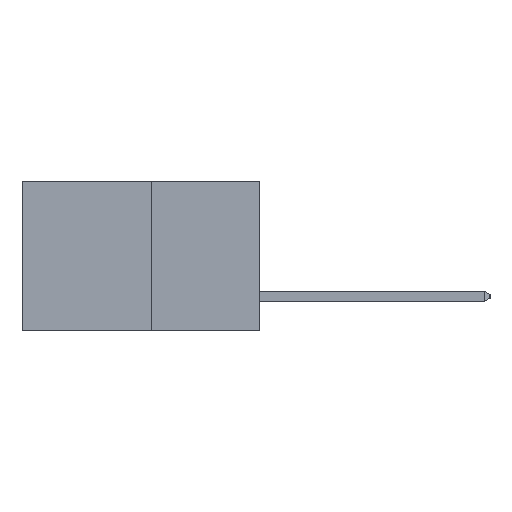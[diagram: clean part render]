
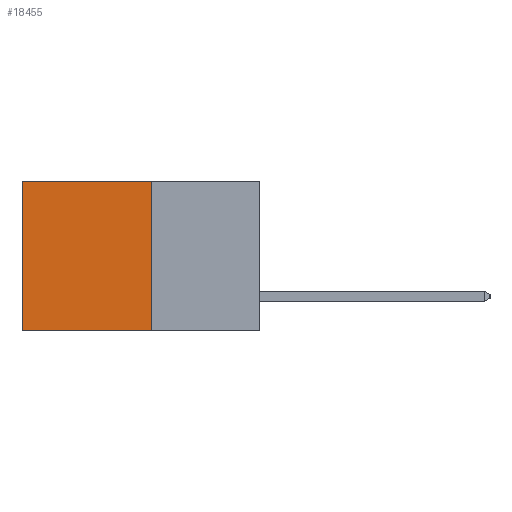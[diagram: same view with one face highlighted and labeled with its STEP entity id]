
A CAD part, left-side view. The second image highlights one B-rep face of the part: STEP entity #18455.
In plain terms, the highlighted planar face has unit normal (-1, 0, 0).
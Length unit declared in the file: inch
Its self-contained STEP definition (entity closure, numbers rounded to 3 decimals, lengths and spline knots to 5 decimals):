
#78 = ORIENTED_EDGE ( 'NONE', *, *, #591, .F. ) ;
#591 = EDGE_CURVE ( 'NONE', #16382, #14361, #10443, .T. ) ;
#1503 = FACE_OUTER_BOUND ( 'NONE', #6174, .T. ) ;
#1516 = CARTESIAN_POINT ( 'NONE',  ( 0.277, 0.27, -0.37 ) ) ;
#1697 = VECTOR ( 'NONE', #2578, 39.37008 ) ;
#2236 = DIRECTION ( 'NONE',  ( 1., 0., 0. ) ) ;
#2578 = DIRECTION ( 'NONE',  ( 0., 0., -1. ) ) ;
#2659 = VECTOR ( 'NONE', #8415, 39.37008 ) ;
#2939 = ORIENTED_EDGE ( 'NONE', *, *, #18609, .F. ) ;
#3146 = LINE ( 'NONE', #12654, #2659 ) ;
#3270 = DIRECTION ( 'NONE',  ( 0., 1., 0. ) ) ;
#3300 = VERTEX_POINT ( 'NONE', #18656 ) ;
#4979 = CARTESIAN_POINT ( 'NONE',  ( 0.277, 0.59, -0.37 ) ) ;
#6075 = LINE ( 'NONE', #18608, #1697 ) ;
#6174 = EDGE_LOOP ( 'NONE', ( #11045, #2939, #78, #15120 ) ) ;
#6550 = VECTOR ( 'NONE', #12598, 39.37008 ) ;
#6616 = PLANE ( 'NONE',  #12386 ) ;
#8415 = DIRECTION ( 'NONE',  ( 0., 1., 0. ) ) ;
#8500 = CARTESIAN_POINT ( 'NONE',  ( 0.277, 0.27, 0. ) ) ;
#10443 = LINE ( 'NONE', #1516, #6550 ) ;
#10547 = CARTESIAN_POINT ( 'NONE',  ( 0.277, 0.27, 0. ) ) ;
#10980 = CARTESIAN_POINT ( 'NONE',  ( 0.277, 0.27, -0.37 ) ) ;
#11045 = ORIENTED_EDGE ( 'NONE', *, *, #11348, .T. ) ;
#11348 = EDGE_CURVE ( 'NONE', #3300, #17337, #6075, .T. ) ;
#12386 = AXIS2_PLACEMENT_3D ( 'NONE', #10980, #2236, #12401 ) ;
#12401 = DIRECTION ( 'NONE',  ( 0., 0., -1. ) ) ;
#12512 = CARTESIAN_POINT ( 'NONE',  ( 0.277, 0.27, -0.37 ) ) ;
#12598 = DIRECTION ( 'NONE',  ( 0., 0., -1. ) ) ;
#12654 = CARTESIAN_POINT ( 'NONE',  ( 0.277, 0.27, -0.37 ) ) ;
#13647 = LINE ( 'NONE', #10547, #17108 ) ;
#14112 = EDGE_CURVE ( 'NONE', #16382, #3300, #13647, .T. ) ;
#14361 = VERTEX_POINT ( 'NONE', #12512 ) ;
#15120 = ORIENTED_EDGE ( 'NONE', *, *, #14112, .T. ) ;
#16382 = VERTEX_POINT ( 'NONE', #8500 ) ;
#17108 = VECTOR ( 'NONE', #3270, 39.37008 ) ;
#17337 = VERTEX_POINT ( 'NONE', #4979 ) ;
#18455 = ADVANCED_FACE ( 'NONE', ( #1503 ), #6616, .F. ) ;
#18608 = CARTESIAN_POINT ( 'NONE',  ( 0.277, 0.59, -0.37 ) ) ;
#18609 = EDGE_CURVE ( 'NONE', #14361, #17337, #3146, .T. ) ;
#18656 = CARTESIAN_POINT ( 'NONE',  ( 0.277, 0.59, 0. ) ) ;
